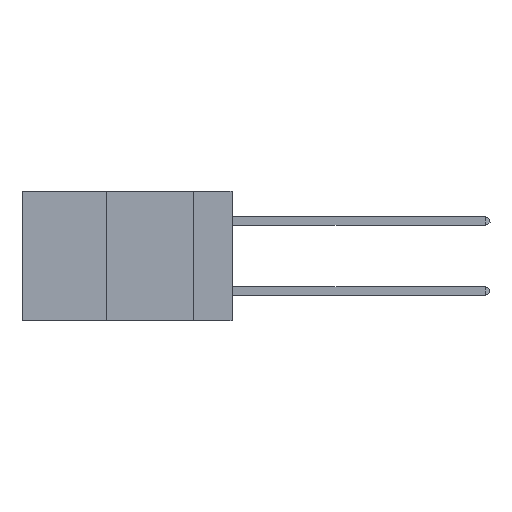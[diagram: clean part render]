
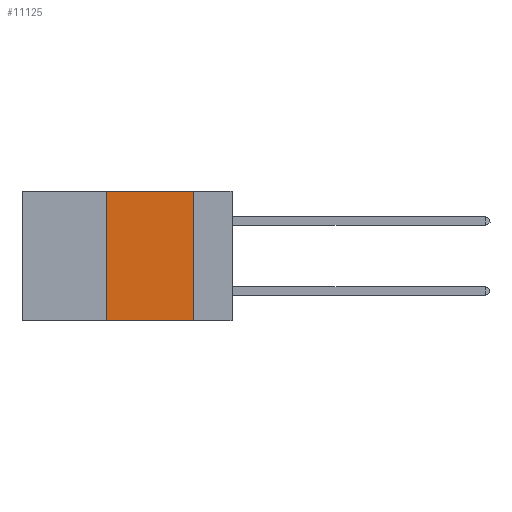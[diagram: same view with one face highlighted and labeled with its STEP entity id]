
A CAD part, left-side view. The second image highlights one B-rep face of the part: STEP entity #11125.
In plain terms, the highlighted planar face has unit normal (-1, 0, 0).
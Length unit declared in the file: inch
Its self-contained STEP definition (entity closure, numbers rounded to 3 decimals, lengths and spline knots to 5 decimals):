
#387 = CARTESIAN_POINT ( 'NONE',  ( 0., 0.6, -0.37 ) ) ;
#626 = LINE ( 'NONE', #3208, #10445 ) ;
#1066 = DIRECTION ( 'NONE',  ( 1., 0., 0. ) ) ;
#1125 = DIRECTION ( 'NONE',  ( 0., 0., -1. ) ) ;
#2338 = VECTOR ( 'NONE', #6187, 39.37008 ) ;
#2967 = ORIENTED_EDGE ( 'NONE', *, *, #10436, .F. ) ;
#3152 = CARTESIAN_POINT ( 'NONE',  ( 0., 0.11, 0. ) ) ;
#3206 = FACE_OUTER_BOUND ( 'NONE', #15135, .T. ) ;
#3208 = CARTESIAN_POINT ( 'NONE',  ( 0., 0.36, 0. ) ) ;
#3408 = VECTOR ( 'NONE', #16077, 39.37008 ) ;
#3611 = LINE ( 'NONE', #387, #3408 ) ;
#3651 = LINE ( 'NONE', #3152, #6969 ) ;
#3736 = PLANE ( 'NONE',  #7965 ) ;
#5219 = EDGE_CURVE ( 'NONE', #13731, #14060, #3611, .T. ) ;
#5664 = LINE ( 'NONE', #14094, #2338 ) ;
#5994 = EDGE_CURVE ( 'NONE', #12605, #6170, #5664, .T. ) ;
#6170 = VERTEX_POINT ( 'NONE', #17069 ) ;
#6187 = DIRECTION ( 'NONE',  ( 0., -1., 0. ) ) ;
#6969 = VECTOR ( 'NONE', #12525, 39.37008 ) ;
#7080 = ORIENTED_EDGE ( 'NONE', *, *, #11688, .F. ) ;
#7965 = AXIS2_PLACEMENT_3D ( 'NONE', #15631, #1066, #1125 ) ;
#10436 = EDGE_CURVE ( 'NONE', #6170, #14060, #3651, .T. ) ;
#10445 = VECTOR ( 'NONE', #12632, 39.37008 ) ;
#11125 = ADVANCED_FACE ( 'NONE', ( #3206 ), #3736, .F. ) ;
#11688 = EDGE_CURVE ( 'NONE', #13731, #12605, #626, .T. ) ;
#12525 = DIRECTION ( 'NONE',  ( 0., 0., -1. ) ) ;
#12605 = VERTEX_POINT ( 'NONE', #14936 ) ;
#12632 = DIRECTION ( 'NONE',  ( 0., 0., 1. ) ) ;
#13731 = VERTEX_POINT ( 'NONE', #15105 ) ;
#14060 = VERTEX_POINT ( 'NONE', #15906 ) ;
#14094 = CARTESIAN_POINT ( 'NONE',  ( 0., 0.6, 0. ) ) ;
#14936 = CARTESIAN_POINT ( 'NONE',  ( 0., 0.36, 0. ) ) ;
#15105 = CARTESIAN_POINT ( 'NONE',  ( 0., 0.36, -0.37 ) ) ;
#15135 = EDGE_LOOP ( 'NONE', ( #2967, #15593, #7080, #15424 ) ) ;
#15424 = ORIENTED_EDGE ( 'NONE', *, *, #5219, .T. ) ;
#15593 = ORIENTED_EDGE ( 'NONE', *, *, #5994, .F. ) ;
#15631 = CARTESIAN_POINT ( 'NONE',  ( 0., 0.6, 0. ) ) ;
#15906 = CARTESIAN_POINT ( 'NONE',  ( 0., 0.11, -0.37 ) ) ;
#16077 = DIRECTION ( 'NONE',  ( 0., -1., 0. ) ) ;
#17069 = CARTESIAN_POINT ( 'NONE',  ( 0., 0.11, 0. ) ) ;
